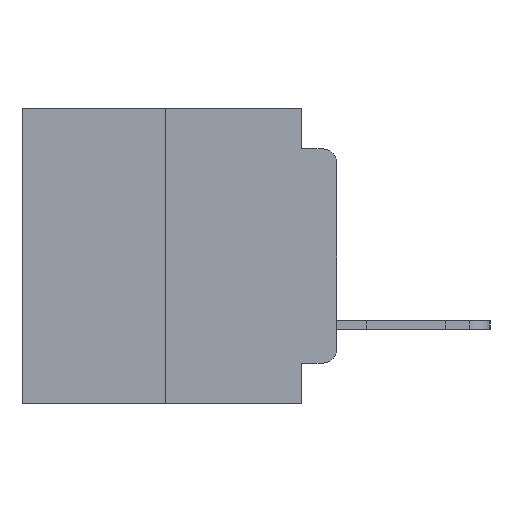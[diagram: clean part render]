
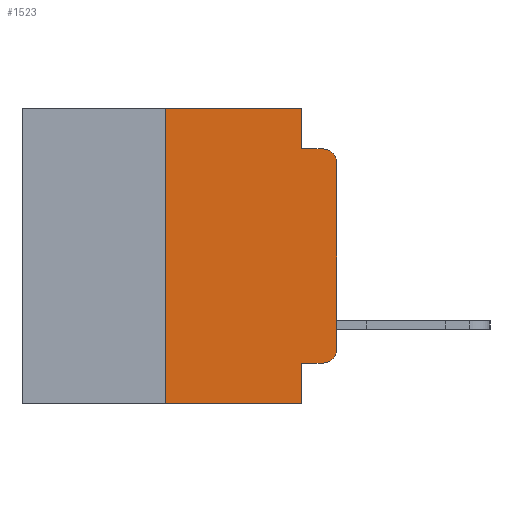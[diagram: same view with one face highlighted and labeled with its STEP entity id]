
A CAD part, left-side view. The second image highlights one B-rep face of the part: STEP entity #1523.
In plain terms, the highlighted planar face has unit normal (-1, 0, 0).
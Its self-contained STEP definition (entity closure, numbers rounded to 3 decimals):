
#667 = VERTEX_POINT ( 'NONE', #20591 ) ;
#1523 = ADVANCED_FACE ( 'NONE', ( #6849 ), #12472, .F. ) ;
#1756 = DIRECTION ( 'NONE',  ( 0., -1., 0. ) ) ;
#2158 = DIRECTION ( 'NONE',  ( -1., 0., 0. ) ) ;
#2247 = CARTESIAN_POINT ( 'NONE',  ( -75.603, 6.35, -5.486 ) ) ;
#2281 = LINE ( 'NONE', #3765, #22219 ) ;
#2429 = EDGE_CURVE ( 'NONE', #6362, #7496, #27503, .T. ) ;
#3765 = CARTESIAN_POINT ( 'NONE',  ( -75.603, 1.295, 0. ) ) ;
#4022 = VERTEX_POINT ( 'NONE', #12814 ) ;
#4538 = CIRCLE ( 'NONE', #24650, 0.508 ) ;
#5072 = LINE ( 'NONE', #28674, #23566 ) ;
#6013 = CARTESIAN_POINT ( 'NONE',  ( -75.603, 0.508, -3.975 ) ) ;
#6200 = VECTOR ( 'NONE', #6928, 1000. ) ;
#6318 = LINE ( 'NONE', #15502, #20917 ) ;
#6362 = VERTEX_POINT ( 'NONE', #6013 ) ;
#6493 = LINE ( 'NONE', #17117, #13247 ) ;
#6619 = VERTEX_POINT ( 'NONE', #11859 ) ;
#6849 = FACE_OUTER_BOUND ( 'NONE', #12194, .T. ) ;
#6856 = DIRECTION ( 'NONE',  ( -1., 0., 0. ) ) ;
#6928 = DIRECTION ( 'NONE',  ( 0., -1., 0. ) ) ;
#7023 = VECTOR ( 'NONE', #19046, 1000. ) ;
#7496 = VERTEX_POINT ( 'NONE', #21968 ) ;
#7708 = ORIENTED_EDGE ( 'NONE', *, *, #26672, .F. ) ;
#7917 = DIRECTION ( 'NONE',  ( 0., 0., -1. ) ) ;
#8086 = AXIS2_PLACEMENT_3D ( 'NONE', #19653, #24098, #7917 ) ;
#8588 = VECTOR ( 'NONE', #26510, 1000. ) ;
#9816 = ORIENTED_EDGE ( 'NONE', *, *, #12397, .F. ) ;
#10340 = VERTEX_POINT ( 'NONE', #20977 ) ;
#10889 = EDGE_CURVE ( 'NONE', #4022, #6362, #16895, .T. ) ;
#11347 = DIRECTION ( 'NONE',  ( 0., 0., -1. ) ) ;
#11859 = CARTESIAN_POINT ( 'NONE',  ( -75.603, 1.295, 5.486 ) ) ;
#11872 = EDGE_CURVE ( 'NONE', #6619, #13001, #6493, .T. ) ;
#12090 = CARTESIAN_POINT ( 'NONE',  ( -75.603, 0.508, 3.975 ) ) ;
#12194 = EDGE_LOOP ( 'NONE', ( #12659, #23914, #12787, #27313, #7708, #19460, #18151, #9816, #13356, #21658 ) ) ;
#12397 = EDGE_CURVE ( 'NONE', #22812, #17255, #24232, .T. ) ;
#12472 = PLANE ( 'NONE',  #8086 ) ;
#12659 = ORIENTED_EDGE ( 'NONE', *, *, #10889, .T. ) ;
#12787 = ORIENTED_EDGE ( 'NONE', *, *, #22635, .T. ) ;
#12814 = CARTESIAN_POINT ( 'NONE',  ( -75.603, 1.295, -3.975 ) ) ;
#13001 = VERTEX_POINT ( 'NONE', #25964 ) ;
#13247 = VECTOR ( 'NONE', #19788, 1000. ) ;
#13356 = ORIENTED_EDGE ( 'NONE', *, *, #14349, .T. ) ;
#14349 = EDGE_CURVE ( 'NONE', #22812, #667, #6318, .T. ) ;
#14456 = CARTESIAN_POINT ( 'NONE',  ( -75.603, 6.35, 5.486 ) ) ;
#15181 = LINE ( 'NONE', #27933, #7023 ) ;
#15502 = CARTESIAN_POINT ( 'NONE',  ( -75.603, 11.684, -5.486 ) ) ;
#16895 = LINE ( 'NONE', #20843, #6200 ) ;
#17117 = CARTESIAN_POINT ( 'NONE',  ( -75.603, 1.295, 0. ) ) ;
#17136 = VERTEX_POINT ( 'NONE', #12090 ) ;
#17255 = VERTEX_POINT ( 'NONE', #14456 ) ;
#17329 = LINE ( 'NONE', #23001, #29456 ) ;
#18151 = ORIENTED_EDGE ( 'NONE', *, *, #18712, .F. ) ;
#18712 = EDGE_CURVE ( 'NONE', #17255, #6619, #17329, .T. ) ;
#18757 = AXIS2_PLACEMENT_3D ( 'NONE', #20487, #2158, #11347 ) ;
#19046 = DIRECTION ( 'NONE',  ( 0., -1., 0. ) ) ;
#19460 = ORIENTED_EDGE ( 'NONE', *, *, #11872, .F. ) ;
#19653 = CARTESIAN_POINT ( 'NONE',  ( -75.603, 11.684, 5.486 ) ) ;
#19714 = EDGE_CURVE ( 'NONE', #4022, #667, #2281, .T. ) ;
#19788 = DIRECTION ( 'NONE',  ( 0., 0., -1. ) ) ;
#20429 = DIRECTION ( 'NONE',  ( 0., -1., 0. ) ) ;
#20487 = CARTESIAN_POINT ( 'NONE',  ( -75.603, 0.508, -3.467 ) ) ;
#20591 = CARTESIAN_POINT ( 'NONE',  ( -75.603, 1.295, -5.486 ) ) ;
#20843 = CARTESIAN_POINT ( 'NONE',  ( -75.603, 1.295, -3.975 ) ) ;
#20917 = VECTOR ( 'NONE', #1756, 1000. ) ;
#20977 = CARTESIAN_POINT ( 'NONE',  ( -75.603, 0., 3.467 ) ) ;
#21658 = ORIENTED_EDGE ( 'NONE', *, *, #19714, .F. ) ;
#21820 = CARTESIAN_POINT ( 'NONE',  ( -75.603, 6.35, -5.486 ) ) ;
#21968 = CARTESIAN_POINT ( 'NONE',  ( -75.603, 0., -3.467 ) ) ;
#21983 = DIRECTION ( 'NONE',  ( 0., 0., -1. ) ) ;
#22219 = VECTOR ( 'NONE', #21983, 1000. ) ;
#22635 = EDGE_CURVE ( 'NONE', #7496, #10340, #5072, .T. ) ;
#22812 = VERTEX_POINT ( 'NONE', #2247 ) ;
#23001 = CARTESIAN_POINT ( 'NONE',  ( -75.603, 11.684, 5.486 ) ) ;
#23566 = VECTOR ( 'NONE', #26988, 1000. ) ;
#23914 = ORIENTED_EDGE ( 'NONE', *, *, #2429, .T. ) ;
#24098 = DIRECTION ( 'NONE',  ( 1., 0., 0. ) ) ;
#24232 = LINE ( 'NONE', #21820, #8588 ) ;
#24650 = AXIS2_PLACEMENT_3D ( 'NONE', #27492, #6856, #27297 ) ;
#25761 = EDGE_CURVE ( 'NONE', #10340, #17136, #4538, .T. ) ;
#25964 = CARTESIAN_POINT ( 'NONE',  ( -75.603, 1.295, 3.975 ) ) ;
#26510 = DIRECTION ( 'NONE',  ( 0., 0., 1. ) ) ;
#26672 = EDGE_CURVE ( 'NONE', #13001, #17136, #15181, .T. ) ;
#26988 = DIRECTION ( 'NONE',  ( 0., 0., 1. ) ) ;
#27297 = DIRECTION ( 'NONE',  ( 0., 0., -1. ) ) ;
#27313 = ORIENTED_EDGE ( 'NONE', *, *, #25761, .T. ) ;
#27492 = CARTESIAN_POINT ( 'NONE',  ( -75.603, 0.508, 3.467 ) ) ;
#27503 = CIRCLE ( 'NONE', #18757, 0.508 ) ;
#27933 = CARTESIAN_POINT ( 'NONE',  ( -75.603, 1.295, 3.975 ) ) ;
#28674 = CARTESIAN_POINT ( 'NONE',  ( -75.603, 0., 5.486 ) ) ;
#29456 = VECTOR ( 'NONE', #20429, 1000. ) ;
